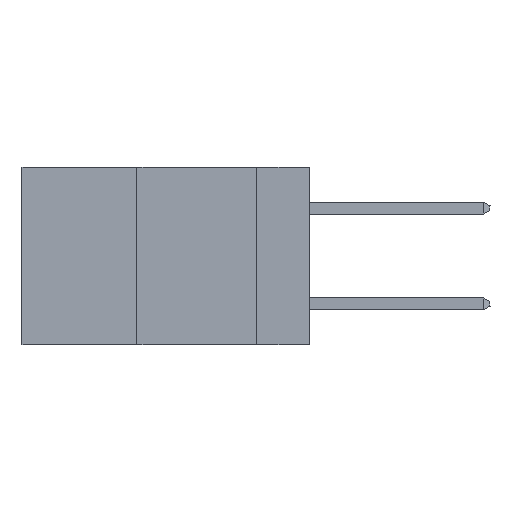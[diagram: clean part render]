
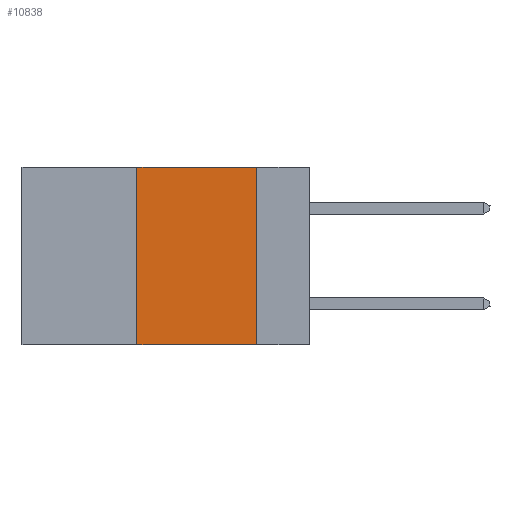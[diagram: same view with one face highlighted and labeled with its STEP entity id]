
A CAD part, left-side view. The second image highlights one B-rep face of the part: STEP entity #10838.
In plain terms, the highlighted planar face has unit normal (-1, 0, 0).
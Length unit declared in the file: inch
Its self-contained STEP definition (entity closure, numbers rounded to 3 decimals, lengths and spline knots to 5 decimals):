
#177 = VECTOR ( 'NONE', #3809, 39.37008 ) ;
#1503 = AXIS2_PLACEMENT_3D ( 'NONE', #2817, #21285, #9086 ) ;
#2214 = FACE_OUTER_BOUND ( 'NONE', #22077, .T. ) ;
#2427 = VERTEX_POINT ( 'NONE', #3652 ) ;
#2817 = CARTESIAN_POINT ( 'NONE',  ( 0., 0.6, 0. ) ) ;
#3652 = CARTESIAN_POINT ( 'NONE',  ( 0., 0.11, -0.37 ) ) ;
#3809 = DIRECTION ( 'NONE',  ( 0., -1., 0. ) ) ;
#4249 = CARTESIAN_POINT ( 'NONE',  ( 0., 0.36, -0.37 ) ) ;
#5640 = DIRECTION ( 'NONE',  ( 0., 0., -1. ) ) ;
#5716 = LINE ( 'NONE', #13423, #14762 ) ;
#5985 = ORIENTED_EDGE ( 'NONE', *, *, #14618, .T. ) ;
#6209 = ORIENTED_EDGE ( 'NONE', *, *, #16661, .F. ) ;
#7001 = PLANE ( 'NONE',  #1503 ) ;
#7192 = CARTESIAN_POINT ( 'NONE',  ( 0., 0.36, 0. ) ) ;
#7221 = LINE ( 'NONE', #23992, #18079 ) ;
#7598 = VERTEX_POINT ( 'NONE', #7192 ) ;
#7811 = CARTESIAN_POINT ( 'NONE',  ( 0., 0.6, 0. ) ) ;
#8616 = ORIENTED_EDGE ( 'NONE', *, *, #21761, .F. ) ;
#9086 = DIRECTION ( 'NONE',  ( 0., 0., -1. ) ) ;
#10838 = ADVANCED_FACE ( 'NONE', ( #2214 ), #7001, .F. ) ;
#13423 = CARTESIAN_POINT ( 'NONE',  ( 0., 0.36, 0. ) ) ;
#13985 = ORIENTED_EDGE ( 'NONE', *, *, #18863, .F. ) ;
#14134 = CARTESIAN_POINT ( 'NONE',  ( 0., 0.6, -0.37 ) ) ;
#14618 = EDGE_CURVE ( 'NONE', #21087, #2427, #21986, .T. ) ;
#14762 = VECTOR ( 'NONE', #15439, 39.37008 ) ;
#14882 = VECTOR ( 'NONE', #15865, 39.37008 ) ;
#15439 = DIRECTION ( 'NONE',  ( 0., 0., 1. ) ) ;
#15865 = DIRECTION ( 'NONE',  ( 0., -1., 0. ) ) ;
#16661 = EDGE_CURVE ( 'NONE', #7598, #20939, #20900, .T. ) ;
#18079 = VECTOR ( 'NONE', #5640, 39.37008 ) ;
#18863 = EDGE_CURVE ( 'NONE', #21087, #7598, #5716, .T. ) ;
#20900 = LINE ( 'NONE', #7811, #14882 ) ;
#20939 = VERTEX_POINT ( 'NONE', #26370 ) ;
#21087 = VERTEX_POINT ( 'NONE', #4249 ) ;
#21285 = DIRECTION ( 'NONE',  ( 1., 0., 0. ) ) ;
#21761 = EDGE_CURVE ( 'NONE', #20939, #2427, #7221, .T. ) ;
#21986 = LINE ( 'NONE', #14134, #177 ) ;
#22077 = EDGE_LOOP ( 'NONE', ( #8616, #6209, #13985, #5985 ) ) ;
#23992 = CARTESIAN_POINT ( 'NONE',  ( 0., 0.11, 0. ) ) ;
#26370 = CARTESIAN_POINT ( 'NONE',  ( 0., 0.11, 0. ) ) ;
